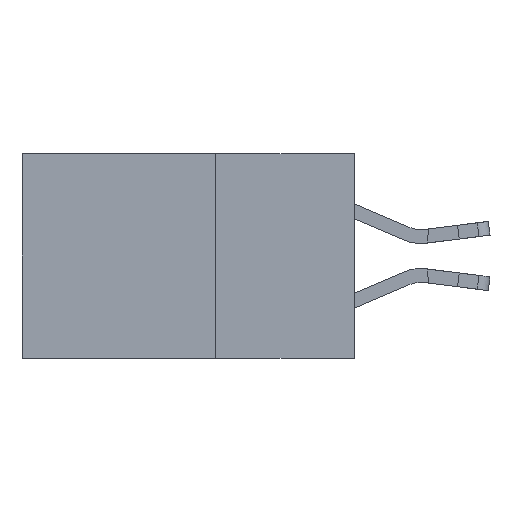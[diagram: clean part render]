
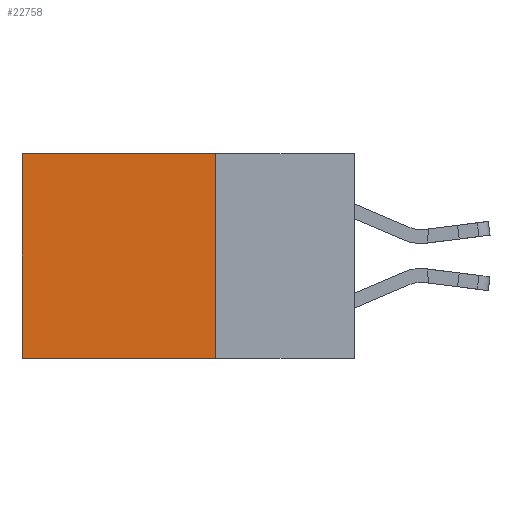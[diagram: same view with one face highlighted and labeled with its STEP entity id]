
A CAD part, left-side view. The second image highlights one B-rep face of the part: STEP entity #22758.
In plain terms, the highlighted planar face has unit normal (-1, 0, 0).
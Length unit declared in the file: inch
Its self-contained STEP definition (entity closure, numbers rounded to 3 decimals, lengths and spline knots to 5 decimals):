
#124 = EDGE_CURVE ( 'NONE', #18417, #15785, #4891, .T. ) ;
#408 = CARTESIAN_POINT ( 'NONE',  ( 0.298, 0.25, -0.37 ) ) ;
#782 = VERTEX_POINT ( 'NONE', #10979 ) ;
#883 = EDGE_CURVE ( 'NONE', #7124, #782, #17861, .T. ) ;
#1207 = DIRECTION ( 'NONE',  ( 1., 0., 0. ) ) ;
#3297 = EDGE_CURVE ( 'NONE', #782, #15785, #17452, .T. ) ;
#3380 = ORIENTED_EDGE ( 'NONE', *, *, #124, .F. ) ;
#4234 = DIRECTION ( 'NONE',  ( 0., 1., 0. ) ) ;
#4298 = VECTOR ( 'NONE', #4234, 39.37008 ) ;
#4891 = LINE ( 'NONE', #5561, #4298 ) ;
#5213 = LINE ( 'NONE', #18074, #19681 ) ;
#5561 = CARTESIAN_POINT ( 'NONE',  ( 0.298, 0.25, -0.37 ) ) ;
#6942 = ORIENTED_EDGE ( 'NONE', *, *, #883, .T. ) ;
#7124 = VERTEX_POINT ( 'NONE', #21056 ) ;
#10082 = EDGE_LOOP ( 'NONE', ( #18393, #3380, #23476, #6942 ) ) ;
#10432 = FACE_OUTER_BOUND ( 'NONE', #10082, .T. ) ;
#10567 = CARTESIAN_POINT ( 'NONE',  ( 0.298, 0.6, -0.37 ) ) ;
#10979 = CARTESIAN_POINT ( 'NONE',  ( 0.298, 0.6, 0. ) ) ;
#12658 = PLANE ( 'NONE',  #19793 ) ;
#14467 = CARTESIAN_POINT ( 'NONE',  ( 0.298, 0.25, 0. ) ) ;
#14547 = DIRECTION ( 'NONE',  ( 0., 0., -1. ) ) ;
#15785 = VERTEX_POINT ( 'NONE', #10567 ) ;
#17452 = LINE ( 'NONE', #20840, #22448 ) ;
#17575 = CARTESIAN_POINT ( 'NONE',  ( 0.298, 0.25, 0. ) ) ;
#17861 = LINE ( 'NONE', #17575, #22268 ) ;
#18074 = CARTESIAN_POINT ( 'NONE',  ( 0.298, 0.25, 0. ) ) ;
#18393 = ORIENTED_EDGE ( 'NONE', *, *, #3297, .T. ) ;
#18417 = VERTEX_POINT ( 'NONE', #408 ) ;
#19681 = VECTOR ( 'NONE', #20040, 39.37008 ) ;
#19793 = AXIS2_PLACEMENT_3D ( 'NONE', #14467, #1207, #14547 ) ;
#20040 = DIRECTION ( 'NONE',  ( 0., 0., -1. ) ) ;
#20152 = EDGE_CURVE ( 'NONE', #7124, #18417, #5213, .T. ) ;
#20750 = DIRECTION ( 'NONE',  ( 0., 0., -1. ) ) ;
#20840 = CARTESIAN_POINT ( 'NONE',  ( 0.298, 0.6, 0. ) ) ;
#21056 = CARTESIAN_POINT ( 'NONE',  ( 0.298, 0.25, 0. ) ) ;
#22268 = VECTOR ( 'NONE', #22580, 39.37008 ) ;
#22448 = VECTOR ( 'NONE', #20750, 39.37008 ) ;
#22580 = DIRECTION ( 'NONE',  ( 0., 1., 0. ) ) ;
#22758 = ADVANCED_FACE ( 'NONE', ( #10432 ), #12658, .F. ) ;
#23476 = ORIENTED_EDGE ( 'NONE', *, *, #20152, .F. ) ;
